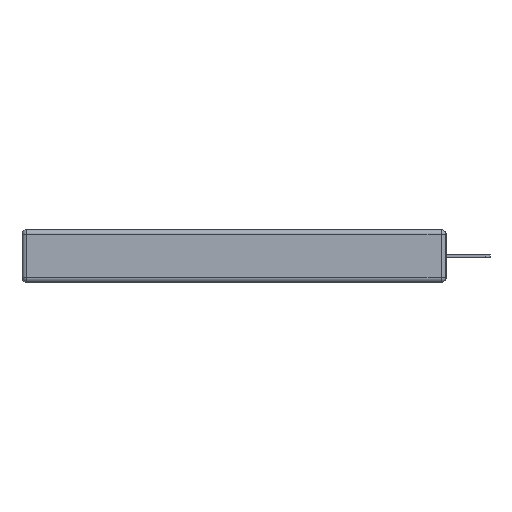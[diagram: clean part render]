
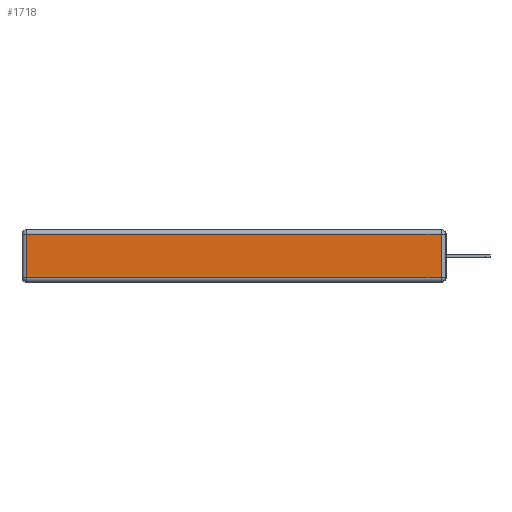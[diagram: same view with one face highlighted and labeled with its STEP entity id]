
A CAD part, left-side view. The second image highlights one B-rep face of the part: STEP entity #1718.
In plain terms, the highlighted planar face has unit normal (-1, 0, 0).
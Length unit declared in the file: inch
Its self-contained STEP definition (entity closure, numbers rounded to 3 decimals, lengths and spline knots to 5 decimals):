
#12 = DIRECTION ( 'NONE',  ( 0., 1., 0. ) ) ;
#1012 = PLANE ( 'NONE',  #8462 ) ;
#1718 = ADVANCED_FACE ( 'NONE', ( #2432 ), #1012, .T. ) ;
#1887 = ORIENTED_EDGE ( 'NONE', *, *, #10383, .T. ) ;
#2069 = VERTEX_POINT ( 'NONE', #11585 ) ;
#2340 = EDGE_CURVE ( 'NONE', #17135, #16097, #3154, .T. ) ;
#2432 = FACE_OUTER_BOUND ( 'NONE', #9373, .T. ) ;
#2602 = DIRECTION ( 'NONE',  ( -1., 0., 0. ) ) ;
#2936 = EDGE_CURVE ( 'NONE', #2069, #17135, #3872, .T. ) ;
#3154 = LINE ( 'NONE', #16104, #5422 ) ;
#3872 = LINE ( 'NONE', #13165, #4868 ) ;
#4043 = CARTESIAN_POINT ( 'NONE',  ( 0., 2.72, -0.03 ) ) ;
#4703 = VECTOR ( 'NONE', #10461, 39.37008 ) ;
#4868 = VECTOR ( 'NONE', #12, 39.37008 ) ;
#5422 = VECTOR ( 'NONE', #5931, 39.37008 ) ;
#5536 = LINE ( 'NONE', #6671, #5991 ) ;
#5931 = DIRECTION ( 'NONE',  ( 0., 0., -1. ) ) ;
#5991 = VECTOR ( 'NONE', #9363, 39.37008 ) ;
#6671 = CARTESIAN_POINT ( 'NONE',  ( 0., 0.03, -0.343 ) ) ;
#8462 = AXIS2_PLACEMENT_3D ( 'NONE', #15725, #2602, #16846 ) ;
#8991 = LINE ( 'NONE', #16872, #4703 ) ;
#9200 = ORIENTED_EDGE ( 'NONE', *, *, #2936, .T. ) ;
#9363 = DIRECTION ( 'NONE',  ( 0., 0., 1. ) ) ;
#9373 = EDGE_LOOP ( 'NONE', ( #9865, #1887, #9200, #13299 ) ) ;
#9735 = VERTEX_POINT ( 'NONE', #13802 ) ;
#9865 = ORIENTED_EDGE ( 'NONE', *, *, #13511, .T. ) ;
#10383 = EDGE_CURVE ( 'NONE', #9735, #2069, #5536, .T. ) ;
#10461 = DIRECTION ( 'NONE',  ( 0., -1., 0. ) ) ;
#11585 = CARTESIAN_POINT ( 'NONE',  ( 0., 0.03, -0.03 ) ) ;
#13165 = CARTESIAN_POINT ( 'NONE',  ( 0., 2.75, -0.03 ) ) ;
#13203 = CARTESIAN_POINT ( 'NONE',  ( 0., 2.72, -0.313 ) ) ;
#13299 = ORIENTED_EDGE ( 'NONE', *, *, #2340, .T. ) ;
#13511 = EDGE_CURVE ( 'NONE', #16097, #9735, #8991, .T. ) ;
#13802 = CARTESIAN_POINT ( 'NONE',  ( 0., 0.03, -0.313 ) ) ;
#15725 = CARTESIAN_POINT ( 'NONE',  ( 0., 0., -0.343 ) ) ;
#16097 = VERTEX_POINT ( 'NONE', #13203 ) ;
#16104 = CARTESIAN_POINT ( 'NONE',  ( 0., 2.72, -0.343 ) ) ;
#16846 = DIRECTION ( 'NONE',  ( 0., 0., 1. ) ) ;
#16872 = CARTESIAN_POINT ( 'NONE',  ( 0., 0., -0.313 ) ) ;
#17135 = VERTEX_POINT ( 'NONE', #4043 ) ;
